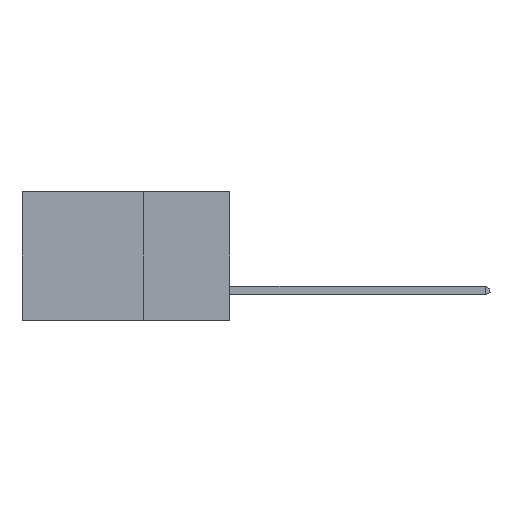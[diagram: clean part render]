
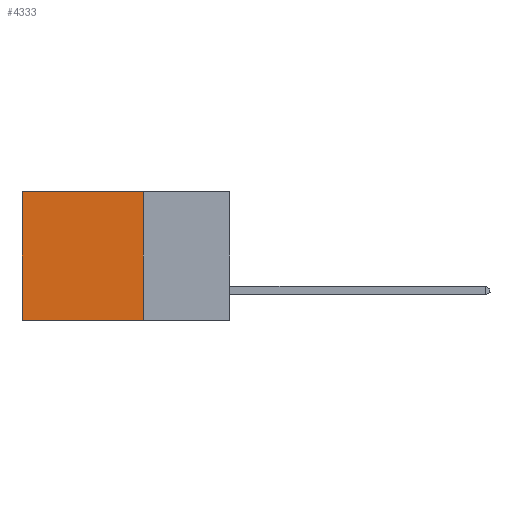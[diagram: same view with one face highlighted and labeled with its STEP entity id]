
A CAD part, left-side view. The second image highlights one B-rep face of the part: STEP entity #4333.
In plain terms, the highlighted planar face has unit normal (-1, 0, 0).
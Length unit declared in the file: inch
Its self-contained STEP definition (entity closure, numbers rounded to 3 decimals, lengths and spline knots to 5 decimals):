
#25 = VECTOR ( 'NONE', #18759, 39.37008 ) ;
#763 = EDGE_CURVE ( 'NONE', #6897, #7331, #6246, .T. ) ;
#975 = EDGE_CURVE ( 'NONE', #12800, #7331, #19919, .T. ) ;
#1099 = EDGE_LOOP ( 'NONE', ( #9770, #5938, #1623, #6349 ) ) ;
#1277 = VERTEX_POINT ( 'NONE', #17957 ) ;
#1623 = ORIENTED_EDGE ( 'NONE', *, *, #14223, .F. ) ;
#2135 = FACE_OUTER_BOUND ( 'NONE', #1099, .T. ) ;
#3573 = CARTESIAN_POINT ( 'NONE',  ( 0.298, 0.6, -0.37 ) ) ;
#3628 = DIRECTION ( 'NONE',  ( 0., 0., -1. ) ) ;
#4333 = ADVANCED_FACE ( 'NONE', ( #2135 ), #18889, .F. ) ;
#5259 = DIRECTION ( 'NONE',  ( 0., 0., -1. ) ) ;
#5752 = VECTOR ( 'NONE', #8205, 39.37008 ) ;
#5938 = ORIENTED_EDGE ( 'NONE', *, *, #975, .F. ) ;
#6017 = LINE ( 'NONE', #6606, #5752 ) ;
#6246 = LINE ( 'NONE', #11906, #18689 ) ;
#6349 = ORIENTED_EDGE ( 'NONE', *, *, #16446, .T. ) ;
#6606 = CARTESIAN_POINT ( 'NONE',  ( 0.298, 0.25, 0. ) ) ;
#6748 = CARTESIAN_POINT ( 'NONE',  ( 0.298, 0.25, 0. ) ) ;
#6897 = VERTEX_POINT ( 'NONE', #18551 ) ;
#7331 = VERTEX_POINT ( 'NONE', #3573 ) ;
#8205 = DIRECTION ( 'NONE',  ( 0., 1., 0. ) ) ;
#9770 = ORIENTED_EDGE ( 'NONE', *, *, #763, .T. ) ;
#10698 = CARTESIAN_POINT ( 'NONE',  ( 0.298, 0.25, -0.37 ) ) ;
#11906 = CARTESIAN_POINT ( 'NONE',  ( 0.298, 0.6, 0. ) ) ;
#12333 = AXIS2_PLACEMENT_3D ( 'NONE', #18819, #14080, #20484 ) ;
#12430 = VECTOR ( 'NONE', #3628, 39.37008 ) ;
#12800 = VERTEX_POINT ( 'NONE', #10698 ) ;
#13949 = CARTESIAN_POINT ( 'NONE',  ( 0.298, 0.25, -0.37 ) ) ;
#14080 = DIRECTION ( 'NONE',  ( 1., 0., 0. ) ) ;
#14223 = EDGE_CURVE ( 'NONE', #1277, #12800, #14958, .T. ) ;
#14958 = LINE ( 'NONE', #6748, #12430 ) ;
#16446 = EDGE_CURVE ( 'NONE', #1277, #6897, #6017, .T. ) ;
#17957 = CARTESIAN_POINT ( 'NONE',  ( 0.298, 0.25, 0. ) ) ;
#18551 = CARTESIAN_POINT ( 'NONE',  ( 0.298, 0.6, 0. ) ) ;
#18689 = VECTOR ( 'NONE', #5259, 39.37008 ) ;
#18759 = DIRECTION ( 'NONE',  ( 0., 1., 0. ) ) ;
#18819 = CARTESIAN_POINT ( 'NONE',  ( 0.298, 0.25, 0. ) ) ;
#18889 = PLANE ( 'NONE',  #12333 ) ;
#19919 = LINE ( 'NONE', #13949, #25 ) ;
#20484 = DIRECTION ( 'NONE',  ( 0., 0., -1. ) ) ;
